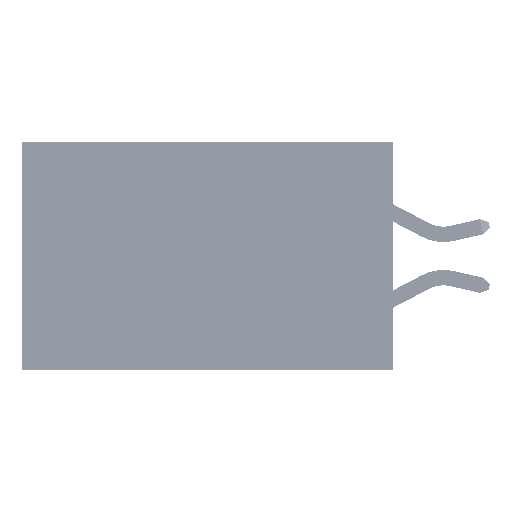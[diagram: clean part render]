
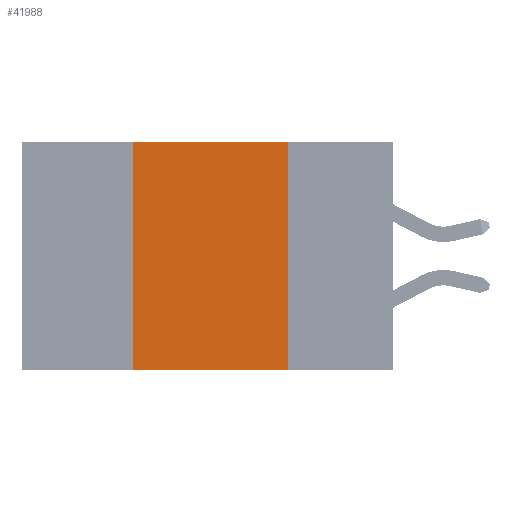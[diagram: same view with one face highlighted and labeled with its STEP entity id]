
A CAD part, left-side view. The second image highlights one B-rep face of the part: STEP entity #41988.
In plain terms, the highlighted planar face has unit normal (-1, 0, 0).
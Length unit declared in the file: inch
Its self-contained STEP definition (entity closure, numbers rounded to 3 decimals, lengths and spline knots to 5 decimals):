
#1022 = CARTESIAN_POINT ( 'NONE',  ( 0., 0.6, -0.37 ) ) ;
#2001 = VECTOR ( 'NONE', #35510, 39.37008 ) ;
#3833 = ORIENTED_EDGE ( 'NONE', *, *, #30080, .T. ) ;
#4438 = CARTESIAN_POINT ( 'NONE',  ( 0., 0.42, 0. ) ) ;
#4698 = AXIS2_PLACEMENT_3D ( 'NONE', #36723, #5747, #28617 ) ;
#5747 = DIRECTION ( 'NONE',  ( 1., 0., 0. ) ) ;
#5871 = VERTEX_POINT ( 'NONE', #8250 ) ;
#6250 = VECTOR ( 'NONE', #43661, 39.37008 ) ;
#8250 = CARTESIAN_POINT ( 'NONE',  ( 0., 0.42, 0. ) ) ;
#8301 = DIRECTION ( 'NONE',  ( 0., 0., 1. ) ) ;
#8738 = VECTOR ( 'NONE', #47024, 39.37008 ) ;
#9328 = LINE ( 'NONE', #11304, #8738 ) ;
#11304 = CARTESIAN_POINT ( 'NONE',  ( 0., 0.6, 0. ) ) ;
#13542 = PLANE ( 'NONE',  #4698 ) ;
#14181 = EDGE_CURVE ( 'NONE', #14796, #27867, #25052, .T. ) ;
#14796 = VERTEX_POINT ( 'NONE', #48151 ) ;
#16486 = ORIENTED_EDGE ( 'NONE', *, *, #45656, .F. ) ;
#20144 = CARTESIAN_POINT ( 'NONE',  ( 0., 0.17, 0. ) ) ;
#20704 = ORIENTED_EDGE ( 'NONE', *, *, #14181, .F. ) ;
#25052 = LINE ( 'NONE', #20144, #2001 ) ;
#27867 = VERTEX_POINT ( 'NONE', #49317 ) ;
#28122 = VECTOR ( 'NONE', #8301, 39.37008 ) ;
#28617 = DIRECTION ( 'NONE',  ( 0., 0., -1. ) ) ;
#30080 = EDGE_CURVE ( 'NONE', #40410, #27867, #37150, .T. ) ;
#32076 = FACE_OUTER_BOUND ( 'NONE', #37828, .T. ) ;
#35510 = DIRECTION ( 'NONE',  ( 0., 0., -1. ) ) ;
#36723 = CARTESIAN_POINT ( 'NONE',  ( 0., 0.6, 0. ) ) ;
#36872 = EDGE_CURVE ( 'NONE', #5871, #14796, #9328, .T. ) ;
#37150 = LINE ( 'NONE', #1022, #6250 ) ;
#37828 = EDGE_LOOP ( 'NONE', ( #20704, #46732, #16486, #3833 ) ) ;
#40410 = VERTEX_POINT ( 'NONE', #44608 ) ;
#41988 = ADVANCED_FACE ( 'NONE', ( #32076 ), #13542, .F. ) ;
#43661 = DIRECTION ( 'NONE',  ( 0., -1., 0. ) ) ;
#44608 = CARTESIAN_POINT ( 'NONE',  ( 0., 0.42, -0.37 ) ) ;
#45656 = EDGE_CURVE ( 'NONE', #40410, #5871, #48050, .T. ) ;
#46732 = ORIENTED_EDGE ( 'NONE', *, *, #36872, .F. ) ;
#47024 = DIRECTION ( 'NONE',  ( 0., -1., 0. ) ) ;
#48050 = LINE ( 'NONE', #4438, #28122 ) ;
#48151 = CARTESIAN_POINT ( 'NONE',  ( 0., 0.17, 0. ) ) ;
#49317 = CARTESIAN_POINT ( 'NONE',  ( 0., 0.17, -0.37 ) ) ;
